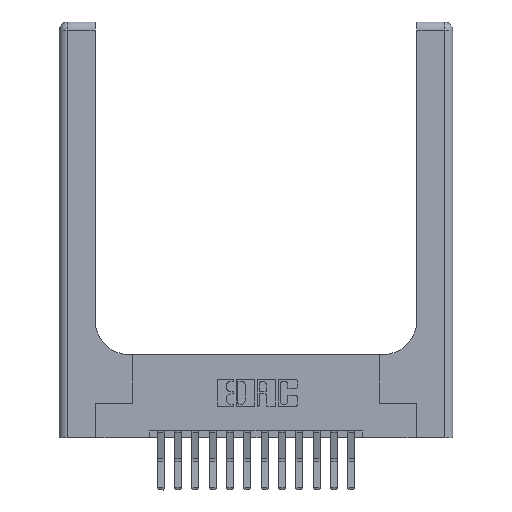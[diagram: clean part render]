
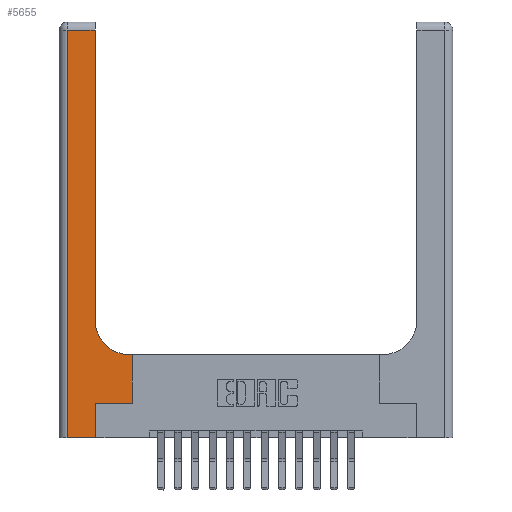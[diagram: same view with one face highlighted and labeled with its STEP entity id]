
A CAD part, top view. The second image highlights one B-rep face of the part: STEP entity #5655.
In plain terms, the highlighted planar face has unit normal (0, 0, 1).
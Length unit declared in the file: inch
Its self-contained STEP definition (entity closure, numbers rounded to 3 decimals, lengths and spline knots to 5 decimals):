
#67 = LINE ( 'NONE', #162, #6696 ) ;
#162 = CARTESIAN_POINT ( 'NONE',  ( 0.26, 3., 0.37 ) ) ;
#240 = VERTEX_POINT ( 'NONE', #5167 ) ;
#259 = EDGE_LOOP ( 'NONE', ( #5225, #701, #9936, #8602, #1180, #1804, #8702, #1238, #10872 ) ) ;
#332 = CARTESIAN_POINT ( 'NONE',  ( 0.26, 0.6, 0.37 ) ) ;
#701 = ORIENTED_EDGE ( 'NONE', *, *, #9926, .T. ) ;
#922 = CARTESIAN_POINT ( 'NONE',  ( 0.06, 2.94, 0.37 ) ) ;
#938 = EDGE_CURVE ( 'NONE', #5477, #14190, #67, .T. ) ;
#994 = CARTESIAN_POINT ( 'NONE',  ( 0.265, 0., 0.37 ) ) ;
#1118 = DIRECTION ( 'NONE',  ( -1., 0., 0. ) ) ;
#1180 = ORIENTED_EDGE ( 'NONE', *, *, #4140, .T. ) ;
#1238 = ORIENTED_EDGE ( 'NONE', *, *, #13094, .T. ) ;
#1537 = LINE ( 'NONE', #1570, #6494 ) ;
#1570 = CARTESIAN_POINT ( 'NONE',  ( 0.06, 3., 0.37 ) ) ;
#1804 = ORIENTED_EDGE ( 'NONE', *, *, #13364, .T. ) ;
#1891 = DIRECTION ( 'NONE',  ( 1., 0., 0. ) ) ;
#2291 = VECTOR ( 'NONE', #1891, 39.37008 ) ;
#2758 = AXIS2_PLACEMENT_3D ( 'NONE', #6083, #7228, #3195 ) ;
#3151 = DIRECTION ( 'NONE',  ( 1., 0., 0. ) ) ;
#3195 = DIRECTION ( 'NONE',  ( 1., 0., 0. ) ) ;
#3272 = VECTOR ( 'NONE', #7239, 39.37008 ) ;
#3857 = VERTEX_POINT ( 'NONE', #5642 ) ;
#3864 = CARTESIAN_POINT ( 'NONE',  ( 0., 3., 0.37 ) ) ;
#4140 = EDGE_CURVE ( 'NONE', #5599, #240, #15280, .T. ) ;
#4523 = VERTEX_POINT ( 'NONE', #922 ) ;
#4706 = CARTESIAN_POINT ( 'NONE',  ( 0., 0., 0.37 ) ) ;
#4862 = VERTEX_POINT ( 'NONE', #11026 ) ;
#5167 = CARTESIAN_POINT ( 'NONE',  ( 0.265, 0.25, 0.37 ) ) ;
#5225 = ORIENTED_EDGE ( 'NONE', *, *, #938, .T. ) ;
#5477 = VERTEX_POINT ( 'NONE', #13950 ) ;
#5497 = LINE ( 'NONE', #8251, #10042 ) ;
#5599 = VERTEX_POINT ( 'NONE', #994 ) ;
#5612 = LINE ( 'NONE', #16352, #2291 ) ;
#5642 = CARTESIAN_POINT ( 'NONE',  ( 0.51, 0.6, 0.37 ) ) ;
#5655 = ADVANCED_FACE ( 'NONE', ( #13806 ), #16789, .F. ) ;
#6083 = CARTESIAN_POINT ( 'NONE',  ( 0.51, 0.85, 0.37 ) ) ;
#6257 = CARTESIAN_POINT ( 'NONE',  ( 0.26, 2.94, 0.37 ) ) ;
#6475 = CARTESIAN_POINT ( 'NONE',  ( 0.528, 0.25, 0.37 ) ) ;
#6494 = VECTOR ( 'NONE', #10821, 39.37008 ) ;
#6696 = VECTOR ( 'NONE', #7140, 39.37008 ) ;
#7140 = DIRECTION ( 'NONE',  ( 0., 1., 0. ) ) ;
#7228 = DIRECTION ( 'NONE',  ( 0., 0., -1. ) ) ;
#7239 = DIRECTION ( 'NONE',  ( 0., 1., 0. ) ) ;
#7338 = VERTEX_POINT ( 'NONE', #6475 ) ;
#7614 = EDGE_CURVE ( 'NONE', #9064, #5599, #7736, .T. ) ;
#7736 = LINE ( 'NONE', #4706, #14388 ) ;
#8251 = CARTESIAN_POINT ( 'NONE',  ( 0., 2.94, 0.37 ) ) ;
#8488 = DIRECTION ( 'NONE',  ( 0., 0., -1. ) ) ;
#8602 = ORIENTED_EDGE ( 'NONE', *, *, #7614, .T. ) ;
#8702 = ORIENTED_EDGE ( 'NONE', *, *, #15168, .T. ) ;
#8924 = VECTOR ( 'NONE', #13423, 39.37008 ) ;
#9064 = VERTEX_POINT ( 'NONE', #16369 ) ;
#9100 = CIRCLE ( 'NONE', #2758, 0.25 ) ;
#9926 = EDGE_CURVE ( 'NONE', #14190, #4523, #5497, .T. ) ;
#9936 = ORIENTED_EDGE ( 'NONE', *, *, #16593, .T. ) ;
#10042 = VECTOR ( 'NONE', #12319, 39.37008 ) ;
#10286 = LINE ( 'NONE', #12970, #12576 ) ;
#10504 = DIRECTION ( 'NONE',  ( 0., 1., 0. ) ) ;
#10821 = DIRECTION ( 'NONE',  ( 0., -1., 0. ) ) ;
#10872 = ORIENTED_EDGE ( 'NONE', *, *, #14007, .T. ) ;
#11026 = CARTESIAN_POINT ( 'NONE',  ( 0.528, 0.6, 0.37 ) ) ;
#12319 = DIRECTION ( 'NONE',  ( -1., 0., 0. ) ) ;
#12576 = VECTOR ( 'NONE', #10504, 39.37008 ) ;
#12832 = CARTESIAN_POINT ( 'NONE',  ( 0.265, 0., 0.37 ) ) ;
#12970 = CARTESIAN_POINT ( 'NONE',  ( 0.528, 0.25, 0.37 ) ) ;
#13094 = EDGE_CURVE ( 'NONE', #4862, #3857, #13482, .T. ) ;
#13364 = EDGE_CURVE ( 'NONE', #240, #7338, #5612, .T. ) ;
#13423 = DIRECTION ( 'NONE',  ( -1., 0., 0. ) ) ;
#13482 = LINE ( 'NONE', #332, #8924 ) ;
#13806 = FACE_OUTER_BOUND ( 'NONE', #259, .T. ) ;
#13950 = CARTESIAN_POINT ( 'NONE',  ( 0.26, 0.85, 0.37 ) ) ;
#14007 = EDGE_CURVE ( 'NONE', #3857, #5477, #9100, .T. ) ;
#14190 = VERTEX_POINT ( 'NONE', #6257 ) ;
#14388 = VECTOR ( 'NONE', #3151, 39.37008 ) ;
#15168 = EDGE_CURVE ( 'NONE', #7338, #4862, #10286, .T. ) ;
#15280 = LINE ( 'NONE', #12832, #3272 ) ;
#16101 = AXIS2_PLACEMENT_3D ( 'NONE', #3864, #8488, #1118 ) ;
#16352 = CARTESIAN_POINT ( 'NONE',  ( 0.265, 0.25, 0.37 ) ) ;
#16369 = CARTESIAN_POINT ( 'NONE',  ( 0.06, 0., 0.37 ) ) ;
#16593 = EDGE_CURVE ( 'NONE', #4523, #9064, #1537, .T. ) ;
#16789 = PLANE ( 'NONE',  #16101 ) ;
